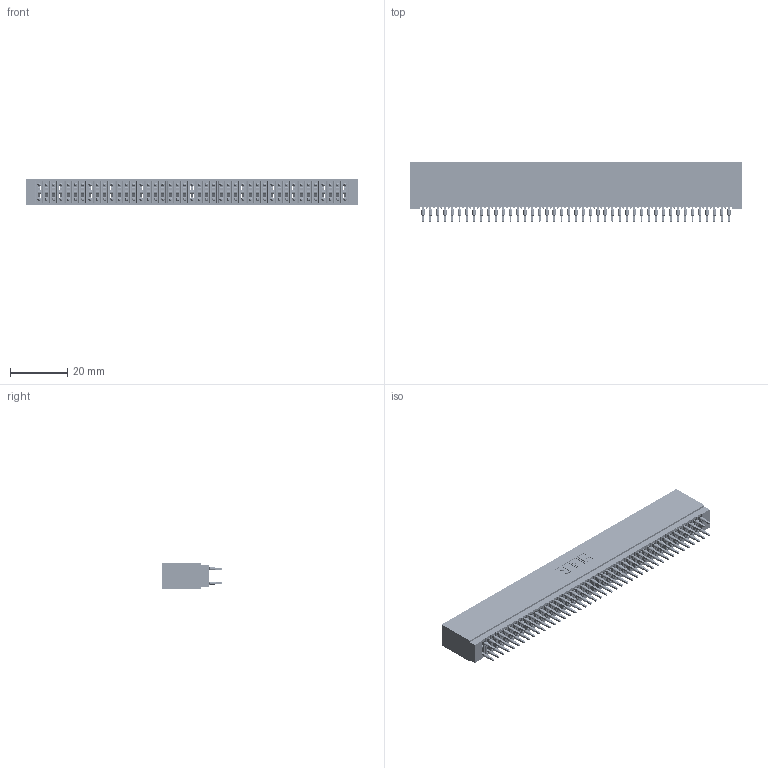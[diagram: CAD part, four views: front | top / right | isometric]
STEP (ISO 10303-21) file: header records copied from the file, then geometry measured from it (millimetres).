
FILE_DESCRIPTION (( 'STEP AP203' ), '1' );
FILE_NAME ('745-086-560-201.STEP', '2026-02-26T22:10:35', ( '' ), ( '' ), 'SwSTEP 2.0', 'SolidWorks 2023', '' );
FILE_SCHEMA (( 'CONFIG_CONTROL_DESIGN' ));
Length unit declared in the file: millimetre
Products named in the file (3): 745-292-001_560; 745-086-560-201; 745 Part_Insulator Option - 01
Assembly tree (87 placements, depth 2):
  745-086-560-201
    745 Part_Insulator Option - 01
    745-292-001_560  x86
Bounding box: 115.82 x 21.22 x 8.89 mm (x, y, z)
Volume: 10743.3 mm3; surface area: 23219.4 mm2
Topology: 87 solids, 87 shells, 8566 faces, 23435 edges, 14878 vertices
Faces by surface type: plane 4441, cylinder 1889, bspline 1720, torus 516
Entity records: 72578 total; most frequent: CARTESIAN_POINT 13093, ORIENTED_EDGE 12530, DIRECTION 10949, EDGE_CURVE 6265, LINE 5817, VECTOR 5817, VERTEX_POINT 3998, AXIS2_PLACEMENT_3D 2566
